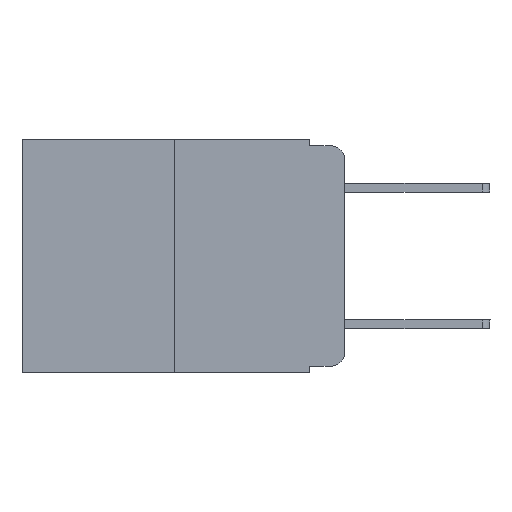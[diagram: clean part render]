
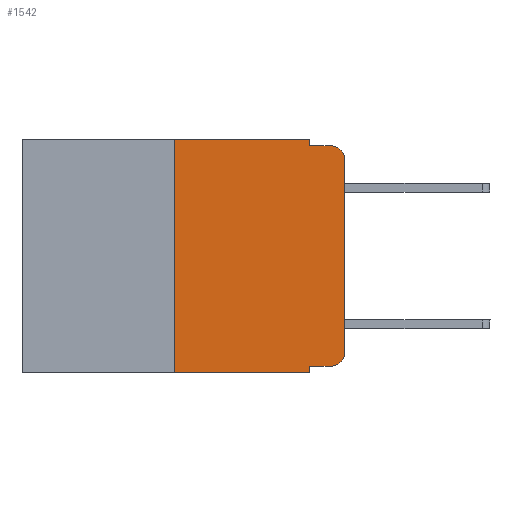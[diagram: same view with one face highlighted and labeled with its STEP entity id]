
A CAD part, left-side view. The second image highlights one B-rep face of the part: STEP entity #1542.
In plain terms, the highlighted planar face has unit normal (-1, 0, 0).
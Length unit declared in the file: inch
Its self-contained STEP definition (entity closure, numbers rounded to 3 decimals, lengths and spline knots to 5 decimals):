
#53 = VERTEX_POINT ( 'NONE', #9293 ) ;
#245 = LINE ( 'NONE', #9893, #2088 ) ;
#358 = EDGE_CURVE ( 'NONE', #1270, #53, #16085, .T. ) ;
#754 = AXIS2_PLACEMENT_3D ( 'NONE', #6939, #2636, #11068 ) ;
#1226 = VECTOR ( 'NONE', #17005, 39.37008 ) ;
#1270 = VERTEX_POINT ( 'NONE', #11946 ) ;
#1542 = ADVANCED_FACE ( 'NONE', ( #8438 ), #13953, .F. ) ;
#1613 = DIRECTION ( 'NONE',  ( 1., 0., 0. ) ) ;
#1701 = DIRECTION ( 'NONE',  ( 0., 0., -1. ) ) ;
#1933 = VERTEX_POINT ( 'NONE', #7475 ) ;
#2012 = DIRECTION ( 'NONE',  ( 0., 0., -1. ) ) ;
#2088 = VECTOR ( 'NONE', #5918, 39.37008 ) ;
#2387 = EDGE_CURVE ( 'NONE', #53, #10873, #7375, .T. ) ;
#2450 = EDGE_LOOP ( 'NONE', ( #14796, #4135, #9781, #10489, #13142, #11470, #2528, #3500, #8504, #2976 ) ) ;
#2528 = ORIENTED_EDGE ( 'NONE', *, *, #2862, .T. ) ;
#2608 = DIRECTION ( 'NONE',  ( -1., 0., 0. ) ) ;
#2636 = DIRECTION ( 'NONE',  ( -1., 0., 0. ) ) ;
#2862 = EDGE_CURVE ( 'NONE', #2884, #7492, #245, .T. ) ;
#2883 = CARTESIAN_POINT ( 'NONE',  ( 0., 0., 0. ) ) ;
#2884 = VERTEX_POINT ( 'NONE', #5746 ) ;
#2900 = EDGE_CURVE ( 'NONE', #2884, #1933, #8617, .T. ) ;
#2976 = ORIENTED_EDGE ( 'NONE', *, *, #4019, .T. ) ;
#3241 = VECTOR ( 'NONE', #8371, 39.37008 ) ;
#3500 = ORIENTED_EDGE ( 'NONE', *, *, #7362, .F. ) ;
#3874 = AXIS2_PLACEMENT_3D ( 'NONE', #9534, #2608, #3964 ) ;
#3964 = DIRECTION ( 'NONE',  ( 0., 0., -1. ) ) ;
#4019 = EDGE_CURVE ( 'NONE', #15499, #6905, #6734, .T. ) ;
#4135 = ORIENTED_EDGE ( 'NONE', *, *, #17174, .T. ) ;
#4463 = LINE ( 'NONE', #11535, #6770 ) ;
#4806 = VERTEX_POINT ( 'NONE', #14002 ) ;
#4976 = CARTESIAN_POINT ( 'NONE',  ( 0., 0.051, 0. ) ) ;
#5564 = CARTESIAN_POINT ( 'NONE',  ( 0., 0.473, 0. ) ) ;
#5746 = CARTESIAN_POINT ( 'NONE',  ( 0., 0.25, -0.343 ) ) ;
#5846 = DIRECTION ( 'NONE',  ( 0., -1., 0. ) ) ;
#5918 = DIRECTION ( 'NONE',  ( 0., -1., 0. ) ) ;
#5971 = LINE ( 'NONE', #17062, #6109 ) ;
#6109 = VECTOR ( 'NONE', #2012, 39.37008 ) ;
#6220 = DIRECTION ( 'NONE',  ( 0., -1., 0. ) ) ;
#6734 = CIRCLE ( 'NONE', #3874, 0.02 ) ;
#6770 = VECTOR ( 'NONE', #12905, 39.37008 ) ;
#6905 = VERTEX_POINT ( 'NONE', #7600 ) ;
#6939 = CARTESIAN_POINT ( 'NONE',  ( 0., 0.02, -0.03 ) ) ;
#7234 = AXIS2_PLACEMENT_3D ( 'NONE', #5564, #1613, #1701 ) ;
#7362 = EDGE_CURVE ( 'NONE', #17230, #7492, #5971, .T. ) ;
#7375 = LINE ( 'NONE', #12864, #8966 ) ;
#7448 = CARTESIAN_POINT ( 'NONE',  ( 0., 0.02, -0.01 ) ) ;
#7475 = CARTESIAN_POINT ( 'NONE',  ( 0., 0.25, 0. ) ) ;
#7492 = VERTEX_POINT ( 'NONE', #12165 ) ;
#7600 = CARTESIAN_POINT ( 'NONE',  ( 0., 0., -0.313 ) ) ;
#7925 = VECTOR ( 'NONE', #6220, 39.37008 ) ;
#8371 = DIRECTION ( 'NONE',  ( 0., 0., 1. ) ) ;
#8438 = FACE_OUTER_BOUND ( 'NONE', #2450, .T. ) ;
#8504 = ORIENTED_EDGE ( 'NONE', *, *, #8680, .T. ) ;
#8617 = LINE ( 'NONE', #11476, #1226 ) ;
#8680 = EDGE_CURVE ( 'NONE', #17230, #15499, #11614, .T. ) ;
#8846 = CARTESIAN_POINT ( 'NONE',  ( 0., 0.051, -0.333 ) ) ;
#8966 = VECTOR ( 'NONE', #5846, 39.37008 ) ;
#9293 = CARTESIAN_POINT ( 'NONE',  ( 0., 0.051, -0.01 ) ) ;
#9534 = CARTESIAN_POINT ( 'NONE',  ( 0., 0.02, -0.313 ) ) ;
#9727 = LINE ( 'NONE', #2883, #3241 ) ;
#9781 = ORIENTED_EDGE ( 'NONE', *, *, #2387, .F. ) ;
#9893 = CARTESIAN_POINT ( 'NONE',  ( 0., 0.473, -0.343 ) ) ;
#10489 = ORIENTED_EDGE ( 'NONE', *, *, #358, .F. ) ;
#10873 = VERTEX_POINT ( 'NONE', #7448 ) ;
#11068 = DIRECTION ( 'NONE',  ( 0., 0., -1. ) ) ;
#11470 = ORIENTED_EDGE ( 'NONE', *, *, #2900, .F. ) ;
#11476 = CARTESIAN_POINT ( 'NONE',  ( 0., 0.25, 0. ) ) ;
#11535 = CARTESIAN_POINT ( 'NONE',  ( 0., 0.473, 0. ) ) ;
#11614 = LINE ( 'NONE', #8846, #7925 ) ;
#11709 = CIRCLE ( 'NONE', #754, 0.02 ) ;
#11946 = CARTESIAN_POINT ( 'NONE',  ( 0., 0.051, 0. ) ) ;
#12122 = EDGE_CURVE ( 'NONE', #6905, #4806, #9727, .T. ) ;
#12165 = CARTESIAN_POINT ( 'NONE',  ( 0., 0.051, -0.343 ) ) ;
#12864 = CARTESIAN_POINT ( 'NONE',  ( 0., 0.051, -0.01 ) ) ;
#12905 = DIRECTION ( 'NONE',  ( 0., -1., 0. ) ) ;
#13142 = ORIENTED_EDGE ( 'NONE', *, *, #14553, .F. ) ;
#13811 = CARTESIAN_POINT ( 'NONE',  ( 0., 0.051, -0.333 ) ) ;
#13953 = PLANE ( 'NONE',  #7234 ) ;
#14002 = CARTESIAN_POINT ( 'NONE',  ( 0., 0., -0.03 ) ) ;
#14553 = EDGE_CURVE ( 'NONE', #1933, #1270, #4463, .T. ) ;
#14648 = VECTOR ( 'NONE', #14813, 39.37008 ) ;
#14796 = ORIENTED_EDGE ( 'NONE', *, *, #12122, .T. ) ;
#14813 = DIRECTION ( 'NONE',  ( 0., 0., -1. ) ) ;
#15499 = VERTEX_POINT ( 'NONE', #17282 ) ;
#16085 = LINE ( 'NONE', #4976, #14648 ) ;
#17005 = DIRECTION ( 'NONE',  ( 0., 0., 1. ) ) ;
#17062 = CARTESIAN_POINT ( 'NONE',  ( 0., 0.051, 0. ) ) ;
#17174 = EDGE_CURVE ( 'NONE', #4806, #10873, #11709, .T. ) ;
#17230 = VERTEX_POINT ( 'NONE', #13811 ) ;
#17282 = CARTESIAN_POINT ( 'NONE',  ( 0., 0.02, -0.333 ) ) ;
